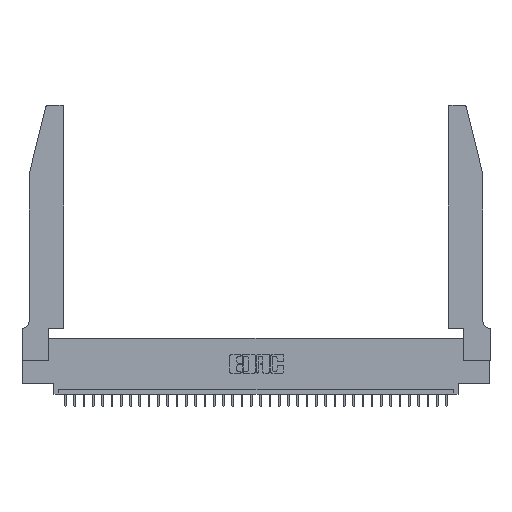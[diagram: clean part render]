
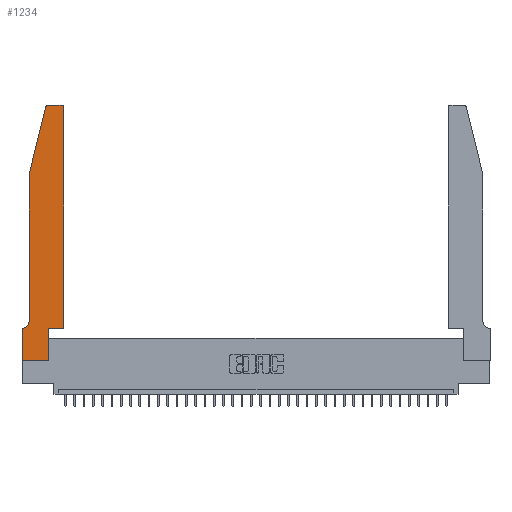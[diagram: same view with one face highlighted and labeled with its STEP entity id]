
A CAD part, top view. The second image highlights one B-rep face of the part: STEP entity #1234.
In plain terms, the highlighted planar face has unit normal (0, 0, 1).
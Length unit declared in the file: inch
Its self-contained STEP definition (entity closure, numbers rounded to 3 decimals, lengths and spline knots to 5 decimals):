
#328 = ORIENTED_EDGE ( 'NONE', *, *, #10092, .T. ) ;
#561 = VERTEX_POINT ( 'NONE', #14018 ) ;
#1145 = DIRECTION ( 'NONE',  ( -0.239, -0.971, 0. ) ) ;
#1234 = ADVANCED_FACE ( 'NONE', ( #25396 ), #13378, .T. ) ;
#1361 = VECTOR ( 'NONE', #14114, 39.37008 ) ;
#1491 = AXIS2_PLACEMENT_3D ( 'NONE', #10603, #8017, #16720 ) ;
#1853 = VECTOR ( 'NONE', #23266, 39.37008 ) ;
#1873 = EDGE_CURVE ( 'NONE', #24069, #11451, #7001, .T. ) ;
#1946 = ORIENTED_EDGE ( 'NONE', *, *, #23673, .T. ) ;
#2600 = EDGE_CURVE ( 'NONE', #19930, #27946, #5991, .T. ) ;
#2691 = ORIENTED_EDGE ( 'NONE', *, *, #29402, .T. ) ;
#2777 = CARTESIAN_POINT ( 'NONE',  ( 0.2865, 0., 0.37 ) ) ;
#3576 = VERTEX_POINT ( 'NONE', #30630 ) ;
#3867 = EDGE_LOOP ( 'NONE', ( #1946, #30840, #11998, #15522, #33590, #328, #35620, #21383, #13803, #21273, #24684, #2691 ) ) ;
#3935 = DIRECTION ( 'NONE',  ( 0., 0., 1. ) ) ;
#4246 = CARTESIAN_POINT ( 'NONE',  ( 0.2865, 0.35, 0.37 ) ) ;
#4346 = CARTESIAN_POINT ( 'NONE',  ( 0.4505, 0.35, 0.37 ) ) ;
#5414 = CARTESIAN_POINT ( 'NONE',  ( 0.0055, 0.42, 0.37 ) ) ;
#5496 = DIRECTION ( 'NONE',  ( -1., 0., 0. ) ) ;
#5575 = EDGE_CURVE ( 'NONE', #19089, #10996, #27789, .T. ) ;
#5601 = DIRECTION ( 'NONE',  ( 1., 0., 0. ) ) ;
#5991 = LINE ( 'NONE', #20785, #15901 ) ;
#6869 = EDGE_CURVE ( 'NONE', #561, #3576, #22773, .T. ) ;
#7001 = LINE ( 'NONE', #7379, #11141 ) ;
#7034 = DIRECTION ( 'NONE',  ( 0., 1., 0. ) ) ;
#7379 = CARTESIAN_POINT ( 'NONE',  ( 0.0755, 2., 0.37 ) ) ;
#7657 = VECTOR ( 'NONE', #7034, 39.37008 ) ;
#8017 = DIRECTION ( 'NONE',  ( 0., 0., 1. ) ) ;
#8235 = VECTOR ( 'NONE', #5496, 39.37008 ) ;
#9098 = CARTESIAN_POINT ( 'NONE',  ( 0.0755, 0.35, 0.37 ) ) ;
#9119 = DIRECTION ( 'NONE',  ( 1., 0., 0. ) ) ;
#10092 = EDGE_CURVE ( 'NONE', #14027, #29044, #34452, .T. ) ;
#10193 = EDGE_CURVE ( 'NONE', #27946, #19089, #33117, .T. ) ;
#10603 = CARTESIAN_POINT ( 'NONE',  ( 0.284, 2.72, 0.37 ) ) ;
#10949 = DIRECTION ( 'NONE',  ( 0., 0., -1. ) ) ;
#10996 = VERTEX_POINT ( 'NONE', #4346 ) ;
#11141 = VECTOR ( 'NONE', #29762, 39.37008 ) ;
#11451 = VERTEX_POINT ( 'NONE', #23233 ) ;
#11998 = ORIENTED_EDGE ( 'NONE', *, *, #17318, .T. ) ;
#13378 = PLANE ( 'NONE',  #29416 ) ;
#13753 = DIRECTION ( 'NONE',  ( 0., 0., 1. ) ) ;
#13803 = ORIENTED_EDGE ( 'NONE', *, *, #10193, .T. ) ;
#13932 = CARTESIAN_POINT ( 'NONE',  ( 0., 0.35, 0.37 ) ) ;
#14018 = CARTESIAN_POINT ( 'NONE',  ( 0.284, 2.75, 0.37 ) ) ;
#14027 = VERTEX_POINT ( 'NONE', #24533 ) ;
#14114 = DIRECTION ( 'NONE',  ( 1., 0., 0. ) ) ;
#14501 = AXIS2_PLACEMENT_3D ( 'NONE', #35033, #3935, #26695 ) ;
#14539 = CARTESIAN_POINT ( 'NONE',  ( 0., 0., 0.37 ) ) ;
#15522 = ORIENTED_EDGE ( 'NONE', *, *, #1873, .T. ) ;
#15812 = CARTESIAN_POINT ( 'NONE',  ( 0., 0.35, 0.37 ) ) ;
#15901 = VECTOR ( 'NONE', #9119, 39.37008 ) ;
#16720 = DIRECTION ( 'NONE',  ( 1., 0., 0. ) ) ;
#17318 = EDGE_CURVE ( 'NONE', #3576, #24069, #34658, .T. ) ;
#18472 = VERTEX_POINT ( 'NONE', #31329 ) ;
#19089 = VERTEX_POINT ( 'NONE', #23703 ) ;
#19250 = VERTEX_POINT ( 'NONE', #22010 ) ;
#19930 = VERTEX_POINT ( 'NONE', #14539 ) ;
#20082 = VECTOR ( 'NONE', #34806, 39.37008 ) ;
#20785 = CARTESIAN_POINT ( 'NONE',  ( 0., 0., 0.37 ) ) ;
#21016 = AXIS2_PLACEMENT_3D ( 'NONE', #5414, #10949, #22251 ) ;
#21273 = ORIENTED_EDGE ( 'NONE', *, *, #5575, .T. ) ;
#21383 = ORIENTED_EDGE ( 'NONE', *, *, #2600, .T. ) ;
#22010 = CARTESIAN_POINT ( 'NONE',  ( 0.4505, 2.72, 0.37 ) ) ;
#22251 = DIRECTION ( 'NONE',  ( -1., 0., 0. ) ) ;
#22334 = LINE ( 'NONE', #23080, #8235 ) ;
#22513 = LINE ( 'NONE', #35072, #1853 ) ;
#22635 = DIRECTION ( 'NONE',  ( 0., 1., 0. ) ) ;
#22773 = CIRCLE ( 'NONE', #1491, 0.03 ) ;
#23080 = CARTESIAN_POINT ( 'NONE',  ( 0.2605, 2.75, 0.37 ) ) ;
#23233 = CARTESIAN_POINT ( 'NONE',  ( 0.0755, 0.42, 0.37 ) ) ;
#23266 = DIRECTION ( 'NONE',  ( 0., -1., 0. ) ) ;
#23376 = CARTESIAN_POINT ( 'NONE',  ( 0.4505, 0.35, 0.37 ) ) ;
#23673 = EDGE_CURVE ( 'NONE', #18472, #561, #22334, .T. ) ;
#23703 = CARTESIAN_POINT ( 'NONE',  ( 0.2865, 0.35, 0.37 ) ) ;
#24069 = VERTEX_POINT ( 'NONE', #24561 ) ;
#24357 = EDGE_CURVE ( 'NONE', #29044, #19930, #22513, .T. ) ;
#24533 = CARTESIAN_POINT ( 'NONE',  ( 0.0055, 0.35, 0.37 ) ) ;
#24561 = CARTESIAN_POINT ( 'NONE',  ( 0.0755, 2., 0.37 ) ) ;
#24684 = ORIENTED_EDGE ( 'NONE', *, *, #36104, .T. ) ;
#25396 = FACE_OUTER_BOUND ( 'NONE', #3867, .T. ) ;
#26695 = DIRECTION ( 'NONE',  ( 1., 0., 0. ) ) ;
#27789 = LINE ( 'NONE', #30948, #1361 ) ;
#27946 = VERTEX_POINT ( 'NONE', #2777 ) ;
#28748 = CIRCLE ( 'NONE', #21016, 0.07 ) ;
#29044 = VERTEX_POINT ( 'NONE', #15812 ) ;
#29075 = CARTESIAN_POINT ( 'NONE',  ( 0.0755, 2., 0.37 ) ) ;
#29402 = EDGE_CURVE ( 'NONE', #19250, #18472, #30451, .T. ) ;
#29416 = AXIS2_PLACEMENT_3D ( 'NONE', #13932, #13753, #5601 ) ;
#29762 = DIRECTION ( 'NONE',  ( 0., -1., 0. ) ) ;
#30451 = CIRCLE ( 'NONE', #14501, 0.03 ) ;
#30630 = CARTESIAN_POINT ( 'NONE',  ( 0.25487, 2.72718, 0.37 ) ) ;
#30801 = EDGE_CURVE ( 'NONE', #11451, #14027, #28748, .T. ) ;
#30840 = ORIENTED_EDGE ( 'NONE', *, *, #6869, .T. ) ;
#30948 = CARTESIAN_POINT ( 'NONE',  ( 0.4505, 0.35, 0.37 ) ) ;
#31329 = CARTESIAN_POINT ( 'NONE',  ( 0.4205, 2.75, 0.37 ) ) ;
#31683 = LINE ( 'NONE', #23376, #34260 ) ;
#33117 = LINE ( 'NONE', #4246, #7657 ) ;
#33590 = ORIENTED_EDGE ( 'NONE', *, *, #30801, .T. ) ;
#34260 = VECTOR ( 'NONE', #22635, 39.37008 ) ;
#34452 = LINE ( 'NONE', #9098, #20082 ) ;
#34658 = LINE ( 'NONE', #29075, #35697 ) ;
#34806 = DIRECTION ( 'NONE',  ( -1., 0., 0. ) ) ;
#35033 = CARTESIAN_POINT ( 'NONE',  ( 0.4205, 2.72, 0.37 ) ) ;
#35072 = CARTESIAN_POINT ( 'NONE',  ( 0., 0., 0.37 ) ) ;
#35620 = ORIENTED_EDGE ( 'NONE', *, *, #24357, .T. ) ;
#35697 = VECTOR ( 'NONE', #1145, 39.37008 ) ;
#36104 = EDGE_CURVE ( 'NONE', #10996, #19250, #31683, .T. ) ;
